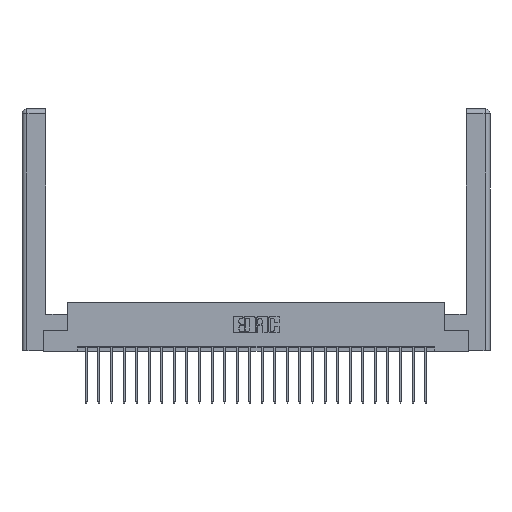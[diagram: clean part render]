
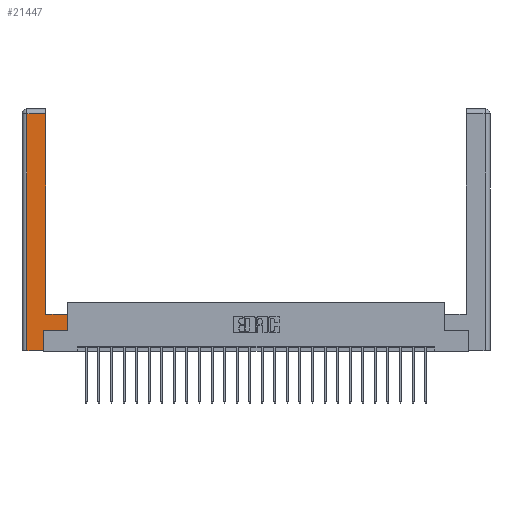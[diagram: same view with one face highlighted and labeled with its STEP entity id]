
A CAD part, top view. The second image highlights one B-rep face of the part: STEP entity #21447.
In plain terms, the highlighted planar face has unit normal (0, 0, 1).
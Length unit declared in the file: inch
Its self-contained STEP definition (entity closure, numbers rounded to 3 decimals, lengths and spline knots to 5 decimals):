
#557 = VERTEX_POINT ( 'NONE', #17868 ) ;
#789 = LINE ( 'NONE', #5583, #4922 ) ;
#812 = ORIENTED_EDGE ( 'NONE', *, *, #17067, .T. ) ;
#1179 = LINE ( 'NONE', #10000, #1795 ) ;
#1620 = CARTESIAN_POINT ( 'NONE',  ( 0.295, 2.94, 0. ) ) ;
#1659 = ORIENTED_EDGE ( 'NONE', *, *, #6082, .T. ) ;
#1795 = VECTOR ( 'NONE', #11701, 39.37008 ) ;
#2152 = CARTESIAN_POINT ( 'NONE',  ( 0.265, 0., 0. ) ) ;
#3620 = VECTOR ( 'NONE', #3695, 39.37008 ) ;
#3641 = CARTESIAN_POINT ( 'NONE',  ( 0.565, 0.245, 0. ) ) ;
#3695 = DIRECTION ( 'NONE',  ( 1., 0., 0. ) ) ;
#3798 = VERTEX_POINT ( 'NONE', #15139 ) ;
#3850 = VECTOR ( 'NONE', #4126, 39.37008 ) ;
#4126 = DIRECTION ( 'NONE',  ( 0., -1., 0. ) ) ;
#4272 = DIRECTION ( 'NONE',  ( -1., 0., 0. ) ) ;
#4844 = DIRECTION ( 'NONE',  ( -1., 0., 0. ) ) ;
#4922 = VECTOR ( 'NONE', #23516, 39.37008 ) ;
#5037 = EDGE_CURVE ( 'NONE', #6809, #9340, #1179, .T. ) ;
#5281 = EDGE_CURVE ( 'NONE', #16464, #557, #5300, .T. ) ;
#5300 = LINE ( 'NONE', #22865, #23613 ) ;
#5583 = CARTESIAN_POINT ( 'NONE',  ( 0.565, 0.45, 0. ) ) ;
#6082 = EDGE_CURVE ( 'NONE', #9938, #11628, #789, .T. ) ;
#6704 = CARTESIAN_POINT ( 'NONE',  ( 0.0615, 0., 0. ) ) ;
#6809 = VERTEX_POINT ( 'NONE', #25616 ) ;
#6833 = ORIENTED_EDGE ( 'NONE', *, *, #5037, .T. ) ;
#8350 = CARTESIAN_POINT ( 'NONE',  ( 0.565, 0.45, 0. ) ) ;
#9319 = VECTOR ( 'NONE', #4844, 39.37008 ) ;
#9340 = VERTEX_POINT ( 'NONE', #1620 ) ;
#9702 = ORIENTED_EDGE ( 'NONE', *, *, #19123, .T. ) ;
#9756 = ORIENTED_EDGE ( 'NONE', *, *, #22832, .T. ) ;
#9938 = VERTEX_POINT ( 'NONE', #3641 ) ;
#9971 = VECTOR ( 'NONE', #21510, 39.37008 ) ;
#10000 = CARTESIAN_POINT ( 'NONE',  ( 0.295, 3., 0. ) ) ;
#10608 = DIRECTION ( 'NONE',  ( 0., 1., 0. ) ) ;
#10726 = VERTEX_POINT ( 'NONE', #6704 ) ;
#11124 = CARTESIAN_POINT ( 'NONE',  ( 0.295, 0.45, 0. ) ) ;
#11628 = VERTEX_POINT ( 'NONE', #8350 ) ;
#11701 = DIRECTION ( 'NONE',  ( 0., 1., 0. ) ) ;
#12194 = CARTESIAN_POINT ( 'NONE',  ( 0.0615, 0., 0. ) ) ;
#12334 = FACE_OUTER_BOUND ( 'NONE', #17055, .T. ) ;
#13104 = AXIS2_PLACEMENT_3D ( 'NONE', #20802, #16562, #4272 ) ;
#13578 = CARTESIAN_POINT ( 'NONE',  ( 0.0615, 2.94, 0. ) ) ;
#13599 = VECTOR ( 'NONE', #17546, 39.37008 ) ;
#13858 = EDGE_CURVE ( 'NONE', #9340, #3798, #17866, .T. ) ;
#14125 = ORIENTED_EDGE ( 'NONE', *, *, #14821, .T. ) ;
#14821 = EDGE_CURVE ( 'NONE', #557, #9938, #24796, .T. ) ;
#15139 = CARTESIAN_POINT ( 'NONE',  ( 0.0615, 2.94, 0. ) ) ;
#15804 = CARTESIAN_POINT ( 'NONE',  ( 0.565, 0.245, 0. ) ) ;
#16377 = PLANE ( 'NONE',  #13104 ) ;
#16464 = VERTEX_POINT ( 'NONE', #2152 ) ;
#16562 = DIRECTION ( 'NONE',  ( 0., 0., -1. ) ) ;
#17055 = EDGE_LOOP ( 'NONE', ( #6833, #18455, #9756, #9702, #21682, #14125, #1659, #812 ) ) ;
#17058 = LINE ( 'NONE', #23377, #13599 ) ;
#17067 = EDGE_CURVE ( 'NONE', #11628, #6809, #24784, .T. ) ;
#17546 = DIRECTION ( 'NONE',  ( 1., 0., 0. ) ) ;
#17866 = LINE ( 'NONE', #13578, #9971 ) ;
#17868 = CARTESIAN_POINT ( 'NONE',  ( 0.265, 0.245, 0. ) ) ;
#18455 = ORIENTED_EDGE ( 'NONE', *, *, #13858, .T. ) ;
#19123 = EDGE_CURVE ( 'NONE', #10726, #16464, #17058, .T. ) ;
#20802 = CARTESIAN_POINT ( 'NONE',  ( 0., 0., 0. ) ) ;
#21447 = ADVANCED_FACE ( 'NONE', ( #12334 ), #16377, .F. ) ;
#21510 = DIRECTION ( 'NONE',  ( -1., 0., 0. ) ) ;
#21682 = ORIENTED_EDGE ( 'NONE', *, *, #5281, .T. ) ;
#22832 = EDGE_CURVE ( 'NONE', #3798, #10726, #25357, .T. ) ;
#22865 = CARTESIAN_POINT ( 'NONE',  ( 0.265, 0.245, 0. ) ) ;
#23377 = CARTESIAN_POINT ( 'NONE',  ( 0.265, 0., 0. ) ) ;
#23516 = DIRECTION ( 'NONE',  ( 0., 1., 0. ) ) ;
#23613 = VECTOR ( 'NONE', #10608, 39.37008 ) ;
#24784 = LINE ( 'NONE', #11124, #9319 ) ;
#24796 = LINE ( 'NONE', #15804, #3620 ) ;
#25357 = LINE ( 'NONE', #12194, #3850 ) ;
#25616 = CARTESIAN_POINT ( 'NONE',  ( 0.295, 0.45, 0. ) ) ;
